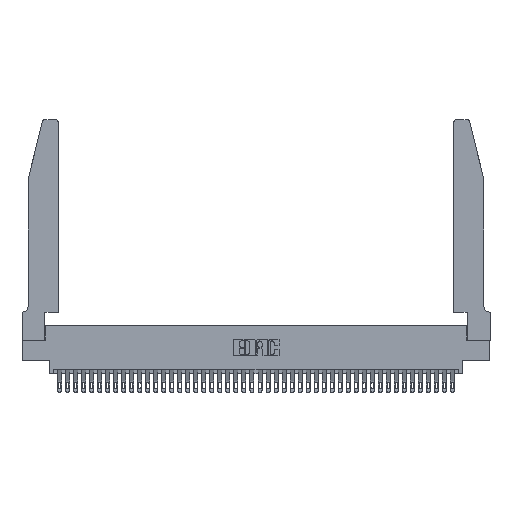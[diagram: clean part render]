
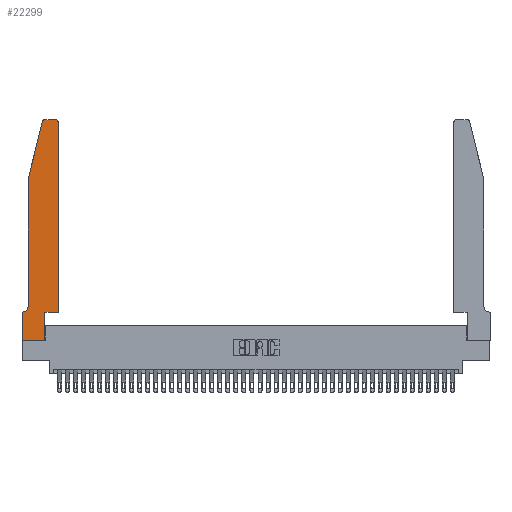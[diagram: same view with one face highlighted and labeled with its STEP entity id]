
A CAD part, top view. The second image highlights one B-rep face of the part: STEP entity #22299.
In plain terms, the highlighted planar face has unit normal (0, 0, 1).
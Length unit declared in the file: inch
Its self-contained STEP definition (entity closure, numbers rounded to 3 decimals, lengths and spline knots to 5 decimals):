
#895 = LINE ( 'NONE', #8902, #21394 ) ;
#985 = CARTESIAN_POINT ( 'NONE',  ( 0.2865, 0., 0.37 ) ) ;
#1435 = EDGE_CURVE ( 'NONE', #6058, #26373, #16965, .T. ) ;
#2074 = EDGE_CURVE ( 'NONE', #21680, #6058, #25372, .T. ) ;
#2577 = ORIENTED_EDGE ( 'NONE', *, *, #28696, .T. ) ;
#2645 = VERTEX_POINT ( 'NONE', #3621 ) ;
#3050 = VECTOR ( 'NONE', #13178, 39.37008 ) ;
#3293 = VERTEX_POINT ( 'NONE', #985 ) ;
#3411 = CARTESIAN_POINT ( 'NONE',  ( 0.284, 2.75, 0.37 ) ) ;
#3420 = VECTOR ( 'NONE', #16057, 39.37008 ) ;
#3493 = CARTESIAN_POINT ( 'NONE',  ( 0.25487, 2.72718, 0.37 ) ) ;
#3621 = CARTESIAN_POINT ( 'NONE',  ( 0., 0., 0.37 ) ) ;
#3680 = CARTESIAN_POINT ( 'NONE',  ( 0.0755, 0.42, 0.37 ) ) ;
#3720 = AXIS2_PLACEMENT_3D ( 'NONE', #27129, #3763, #14005 ) ;
#3763 = DIRECTION ( 'NONE',  ( 0., 0., 1. ) ) ;
#4305 = ORIENTED_EDGE ( 'NONE', *, *, #28110, .T. ) ;
#4589 = VECTOR ( 'NONE', #10681, 39.37008 ) ;
#5050 = AXIS2_PLACEMENT_3D ( 'NONE', #20718, #31044, #34366 ) ;
#5467 = CARTESIAN_POINT ( 'NONE',  ( 0.0755, 2., 0.37 ) ) ;
#6058 = VERTEX_POINT ( 'NONE', #3411 ) ;
#6124 = LINE ( 'NONE', #30577, #8751 ) ;
#6595 = VERTEX_POINT ( 'NONE', #29662 ) ;
#6655 = VECTOR ( 'NONE', #13096, 39.37008 ) ;
#7141 = CARTESIAN_POINT ( 'NONE',  ( 0., 0., 0.37 ) ) ;
#7178 = LINE ( 'NONE', #43225, #3050 ) ;
#8201 = LINE ( 'NONE', #5467, #9843 ) ;
#8751 = VECTOR ( 'NONE', #23535, 39.37008 ) ;
#8846 = CARTESIAN_POINT ( 'NONE',  ( 0.0755, 0.35, 0.37 ) ) ;
#8902 = CARTESIAN_POINT ( 'NONE',  ( 0.0755, 2., 0.37 ) ) ;
#9843 = VECTOR ( 'NONE', #22391, 39.37008 ) ;
#10205 = LINE ( 'NONE', #8846, #3420 ) ;
#10247 = VERTEX_POINT ( 'NONE', #21200 ) ;
#10566 = EDGE_CURVE ( 'NONE', #26373, #14741, #895, .T. ) ;
#10681 = DIRECTION ( 'NONE',  ( 1., 0., 0. ) ) ;
#10792 = DIRECTION ( 'NONE',  ( -1., 0., 0. ) ) ;
#10939 = CARTESIAN_POINT ( 'NONE',  ( 0.0055, 0.42, 0.37 ) ) ;
#13096 = DIRECTION ( 'NONE',  ( 0., -1., 0. ) ) ;
#13178 = DIRECTION ( 'NONE',  ( 1., 0., 0. ) ) ;
#13489 = EDGE_LOOP ( 'NONE', ( #27198, #14223, #18699, #29988, #26093, #16319, #4305, #29490, #42749, #2577, #30562, #40688 ) ) ;
#13918 = CARTESIAN_POINT ( 'NONE',  ( 0., 0.35, 0.37 ) ) ;
#14005 = DIRECTION ( 'NONE',  ( 1., 0., 0. ) ) ;
#14029 = AXIS2_PLACEMENT_3D ( 'NONE', #23213, #39861, #42798 ) ;
#14223 = ORIENTED_EDGE ( 'NONE', *, *, #1435, .T. ) ;
#14741 = VERTEX_POINT ( 'NONE', #34412 ) ;
#15791 = DIRECTION ( 'NONE',  ( 0., 1., 0. ) ) ;
#16057 = DIRECTION ( 'NONE',  ( -1., 0., 0. ) ) ;
#16319 = ORIENTED_EDGE ( 'NONE', *, *, #39763, .T. ) ;
#16691 = LINE ( 'NONE', #7141, #4589 ) ;
#16846 = CARTESIAN_POINT ( 'NONE',  ( 0.0055, 0.35, 0.37 ) ) ;
#16965 = CIRCLE ( 'NONE', #14029, 0.03 ) ;
#17090 = CARTESIAN_POINT ( 'NONE',  ( 0.2605, 2.75, 0.37 ) ) ;
#18699 = ORIENTED_EDGE ( 'NONE', *, *, #10566, .T. ) ;
#19601 = VERTEX_POINT ( 'NONE', #24459 ) ;
#20259 = LINE ( 'NONE', #25843, #34946 ) ;
#20718 = CARTESIAN_POINT ( 'NONE',  ( 0.4205, 2.72, 0.37 ) ) ;
#21200 = CARTESIAN_POINT ( 'NONE',  ( 0.4505, 2.72, 0.37 ) ) ;
#21394 = VECTOR ( 'NONE', #28944, 39.37008 ) ;
#21680 = VERTEX_POINT ( 'NONE', #42528 ) ;
#22299 = ADVANCED_FACE ( 'NONE', ( #29264 ), #40399, .T. ) ;
#22391 = DIRECTION ( 'NONE',  ( 0., -1., 0. ) ) ;
#22785 = VECTOR ( 'NONE', #23754, 39.37008 ) ;
#23213 = CARTESIAN_POINT ( 'NONE',  ( 0.284, 2.72, 0.37 ) ) ;
#23535 = DIRECTION ( 'NONE',  ( 0., 1., 0. ) ) ;
#23578 = VERTEX_POINT ( 'NONE', #13918 ) ;
#23754 = DIRECTION ( 'NONE',  ( -1., 0., 0. ) ) ;
#24459 = CARTESIAN_POINT ( 'NONE',  ( 0.4505, 0.35, 0.37 ) ) ;
#24877 = CIRCLE ( 'NONE', #25290, 0.07 ) ;
#25290 = AXIS2_PLACEMENT_3D ( 'NONE', #10939, #34857, #10792 ) ;
#25372 = LINE ( 'NONE', #17090, #22785 ) ;
#25843 = CARTESIAN_POINT ( 'NONE',  ( 0.2865, 0.35, 0.37 ) ) ;
#26093 = ORIENTED_EDGE ( 'NONE', *, *, #41676, .T. ) ;
#26373 = VERTEX_POINT ( 'NONE', #3493 ) ;
#26473 = EDGE_CURVE ( 'NONE', #10247, #21680, #37766, .T. ) ;
#26769 = CARTESIAN_POINT ( 'NONE',  ( 0., 0., 0.37 ) ) ;
#27129 = CARTESIAN_POINT ( 'NONE',  ( 0., 0.35, 0.37 ) ) ;
#27198 = ORIENTED_EDGE ( 'NONE', *, *, #2074, .T. ) ;
#28094 = VERTEX_POINT ( 'NONE', #16846 ) ;
#28110 = EDGE_CURVE ( 'NONE', #23578, #2645, #39208, .T. ) ;
#28340 = EDGE_CURVE ( 'NONE', #2645, #3293, #16691, .T. ) ;
#28696 = EDGE_CURVE ( 'NONE', #6595, #19601, #7178, .T. ) ;
#28944 = DIRECTION ( 'NONE',  ( -0.239, -0.971, 0. ) ) ;
#29264 = FACE_OUTER_BOUND ( 'NONE', #13489, .T. ) ;
#29490 = ORIENTED_EDGE ( 'NONE', *, *, #28340, .T. ) ;
#29662 = CARTESIAN_POINT ( 'NONE',  ( 0.2865, 0.35, 0.37 ) ) ;
#29988 = ORIENTED_EDGE ( 'NONE', *, *, #38333, .T. ) ;
#30246 = VERTEX_POINT ( 'NONE', #3680 ) ;
#30562 = ORIENTED_EDGE ( 'NONE', *, *, #38582, .T. ) ;
#30577 = CARTESIAN_POINT ( 'NONE',  ( 0.4505, 0.35, 0.37 ) ) ;
#31044 = DIRECTION ( 'NONE',  ( 0., 0., 1. ) ) ;
#34366 = DIRECTION ( 'NONE',  ( 1., 0., 0. ) ) ;
#34412 = CARTESIAN_POINT ( 'NONE',  ( 0.0755, 2., 0.37 ) ) ;
#34857 = DIRECTION ( 'NONE',  ( 0., 0., -1. ) ) ;
#34946 = VECTOR ( 'NONE', #15791, 39.37008 ) ;
#35633 = EDGE_CURVE ( 'NONE', #3293, #6595, #20259, .T. ) ;
#37766 = CIRCLE ( 'NONE', #5050, 0.03 ) ;
#38333 = EDGE_CURVE ( 'NONE', #14741, #30246, #8201, .T. ) ;
#38582 = EDGE_CURVE ( 'NONE', #19601, #10247, #6124, .T. ) ;
#39208 = LINE ( 'NONE', #26769, #6655 ) ;
#39763 = EDGE_CURVE ( 'NONE', #28094, #23578, #10205, .T. ) ;
#39861 = DIRECTION ( 'NONE',  ( 0., 0., 1. ) ) ;
#40399 = PLANE ( 'NONE',  #3720 ) ;
#40688 = ORIENTED_EDGE ( 'NONE', *, *, #26473, .T. ) ;
#41676 = EDGE_CURVE ( 'NONE', #30246, #28094, #24877, .T. ) ;
#42528 = CARTESIAN_POINT ( 'NONE',  ( 0.4205, 2.75, 0.37 ) ) ;
#42749 = ORIENTED_EDGE ( 'NONE', *, *, #35633, .T. ) ;
#42798 = DIRECTION ( 'NONE',  ( 1., 0., 0. ) ) ;
#43225 = CARTESIAN_POINT ( 'NONE',  ( 0.4505, 0.35, 0.37 ) ) ;
